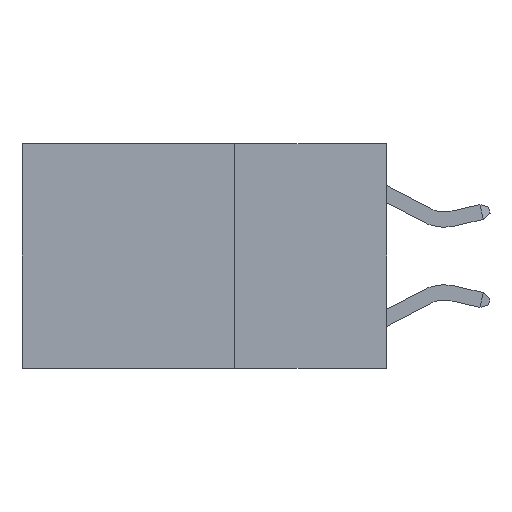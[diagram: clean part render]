
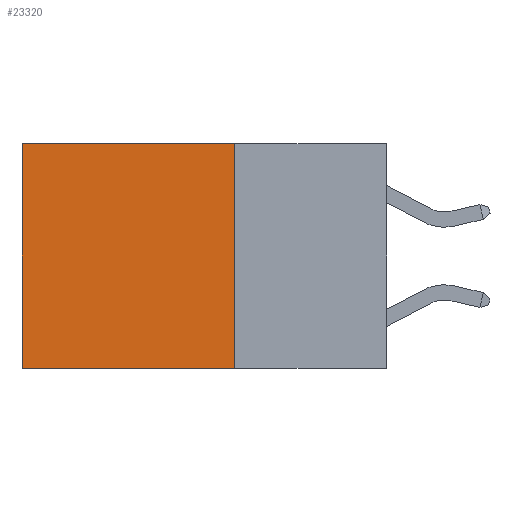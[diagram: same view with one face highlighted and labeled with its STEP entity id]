
A CAD part, left-side view. The second image highlights one B-rep face of the part: STEP entity #23320.
In plain terms, the highlighted planar face has unit normal (-1, 0, 0).
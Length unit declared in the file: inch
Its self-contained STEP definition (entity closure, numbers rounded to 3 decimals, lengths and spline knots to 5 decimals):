
#753 = EDGE_LOOP ( 'NONE', ( #2725, #8792, #25280, #15547 ) ) ;
#1776 = LINE ( 'NONE', #21893, #21813 ) ;
#2725 = ORIENTED_EDGE ( 'NONE', *, *, #5126, .T. ) ;
#3316 = DIRECTION ( 'NONE',  ( 0., 0., -1. ) ) ;
#4144 = CARTESIAN_POINT ( 'NONE',  ( 0.2625, 0.25, 0. ) ) ;
#5126 = EDGE_CURVE ( 'NONE', #11671, #26248, #15839, .T. ) ;
#7416 = VERTEX_POINT ( 'NONE', #15025 ) ;
#7484 = DIRECTION ( 'NONE',  ( 0., 0., -1. ) ) ;
#7735 = CARTESIAN_POINT ( 'NONE',  ( 0.2625, 0.25, 0. ) ) ;
#8291 = DIRECTION ( 'NONE',  ( 0., 0., -1. ) ) ;
#8446 = CARTESIAN_POINT ( 'NONE',  ( 0.2625, 0.25, -0.37 ) ) ;
#8792 = ORIENTED_EDGE ( 'NONE', *, *, #17834, .F. ) ;
#10199 = DIRECTION ( 'NONE',  ( 1., 0., 0. ) ) ;
#10711 = VERTEX_POINT ( 'NONE', #25260 ) ;
#11671 = VERTEX_POINT ( 'NONE', #17968 ) ;
#13895 = EDGE_CURVE ( 'NONE', #7416, #10711, #19989, .T. ) ;
#14516 = VECTOR ( 'NONE', #7484, 39.37008 ) ;
#15025 = CARTESIAN_POINT ( 'NONE',  ( 0.2625, 0.25, 0. ) ) ;
#15547 = ORIENTED_EDGE ( 'NONE', *, *, #25009, .T. ) ;
#15631 = DIRECTION ( 'NONE',  ( 0., 1., 0. ) ) ;
#15839 = LINE ( 'NONE', #24229, #14516 ) ;
#17222 = LINE ( 'NONE', #8446, #23145 ) ;
#17834 = EDGE_CURVE ( 'NONE', #10711, #26248, #17222, .T. ) ;
#17968 = CARTESIAN_POINT ( 'NONE',  ( 0.2625, 0.6, 0. ) ) ;
#19989 = LINE ( 'NONE', #7735, #22626 ) ;
#21464 = CARTESIAN_POINT ( 'NONE',  ( 0.2625, 0.6, -0.37 ) ) ;
#21586 = FACE_OUTER_BOUND ( 'NONE', #753, .T. ) ;
#21813 = VECTOR ( 'NONE', #15631, 39.37008 ) ;
#21893 = CARTESIAN_POINT ( 'NONE',  ( 0.2625, 0.25, 0. ) ) ;
#22318 = AXIS2_PLACEMENT_3D ( 'NONE', #4144, #10199, #8291 ) ;
#22626 = VECTOR ( 'NONE', #3316, 39.37008 ) ;
#22709 = DIRECTION ( 'NONE',  ( 0., 1., 0. ) ) ;
#23145 = VECTOR ( 'NONE', #22709, 39.37008 ) ;
#23320 = ADVANCED_FACE ( 'NONE', ( #21586 ), #24661, .F. ) ;
#24229 = CARTESIAN_POINT ( 'NONE',  ( 0.2625, 0.6, 0. ) ) ;
#24661 = PLANE ( 'NONE',  #22318 ) ;
#25009 = EDGE_CURVE ( 'NONE', #7416, #11671, #1776, .T. ) ;
#25260 = CARTESIAN_POINT ( 'NONE',  ( 0.2625, 0.25, -0.37 ) ) ;
#25280 = ORIENTED_EDGE ( 'NONE', *, *, #13895, .F. ) ;
#26248 = VERTEX_POINT ( 'NONE', #21464 ) ;
